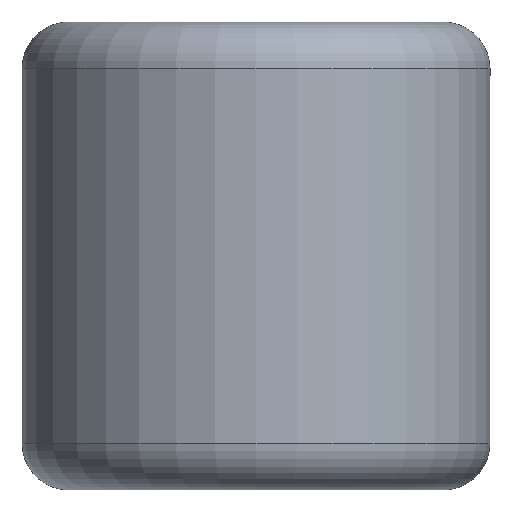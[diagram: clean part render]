
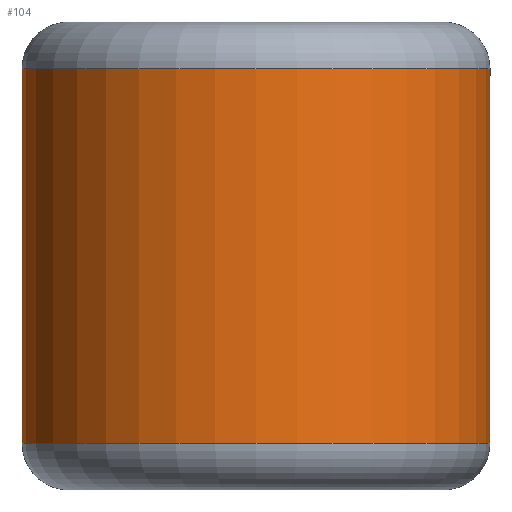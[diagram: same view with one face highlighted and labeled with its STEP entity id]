
A CAD part, left-side view. The second image highlights one B-rep face of the part: STEP entity #104.
In plain terms, the highlighted cylindrical face has radius 5 mm (diameter 10 mm), a partial arc.
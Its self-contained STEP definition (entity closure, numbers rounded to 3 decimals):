
#1 = EDGE_CURVE ( 'NONE', #116, #120, #55, .T. ) ;
#17 = AXIS2_PLACEMENT_3D ( 'NONE', #171, #175, #162 ) ;
#28 = CYLINDRICAL_SURFACE ( 'NONE', #46, 5. ) ;
#30 = EDGE_CURVE ( 'NONE', #116, #189, #185, .T. ) ;
#32 = VECTOR ( 'NONE', #237, 1000. ) ;
#46 = AXIS2_PLACEMENT_3D ( 'NONE', #106, #131, #80 ) ;
#55 = LINE ( 'NONE', #216, #32 ) ;
#56 = EDGE_CURVE ( 'NONE', #110, #120, #75, .T. ) ;
#75 = CIRCLE ( 'NONE', #17, 5. ) ;
#77 = CARTESIAN_POINT ( 'NONE',  ( 0., 10., 4. ) ) ;
#80 = DIRECTION ( 'NONE',  ( 0., 1., 0. ) ) ;
#83 = CARTESIAN_POINT ( 'NONE',  ( 0., 0., -4. ) ) ;
#88 = EDGE_CURVE ( 'NONE', #189, #110, #139, .T. ) ;
#98 = ORIENTED_EDGE ( 'NONE', *, *, #1, .F. ) ;
#100 = ORIENTED_EDGE ( 'NONE', *, *, #56, .T. ) ;
#104 = ADVANCED_FACE ( 'NONE', ( #158 ), #28, .T. ) ;
#106 = CARTESIAN_POINT ( 'NONE',  ( 0., 5., 5. ) ) ;
#109 = DIRECTION ( 'NONE',  ( 0., 0., -1. ) ) ;
#110 = VERTEX_POINT ( 'NONE', #136 ) ;
#114 = ORIENTED_EDGE ( 'NONE', *, *, #30, .T. ) ;
#116 = VERTEX_POINT ( 'NONE', #123 ) ;
#120 = VERTEX_POINT ( 'NONE', #83 ) ;
#123 = CARTESIAN_POINT ( 'NONE',  ( 0., 0., 4. ) ) ;
#127 = CARTESIAN_POINT ( 'NONE',  ( 0., 10., 5. ) ) ;
#131 = DIRECTION ( 'NONE',  ( 0., 0., -1. ) ) ;
#136 = CARTESIAN_POINT ( 'NONE',  ( 0., 10., -4. ) ) ;
#138 = VECTOR ( 'NONE', #109, 1000. ) ;
#139 = LINE ( 'NONE', #127, #138 ) ;
#158 = FACE_OUTER_BOUND ( 'NONE', #239, .T. ) ;
#162 = DIRECTION ( 'NONE',  ( 0., -1., 0. ) ) ;
#171 = CARTESIAN_POINT ( 'NONE',  ( 0., 5., -4. ) ) ;
#175 = DIRECTION ( 'NONE',  ( 0., 0., 1. ) ) ;
#185 = CIRCLE ( 'NONE', #241, 5. ) ;
#189 = VERTEX_POINT ( 'NONE', #77 ) ;
#216 = CARTESIAN_POINT ( 'NONE',  ( 0., 0., 5. ) ) ;
#227 = CARTESIAN_POINT ( 'NONE',  ( 0., 5., 4. ) ) ;
#228 = DIRECTION ( 'NONE',  ( 0., 0., -1. ) ) ;
#229 = ORIENTED_EDGE ( 'NONE', *, *, #88, .T. ) ;
#230 = DIRECTION ( 'NONE',  ( 0., -1., 0. ) ) ;
#237 = DIRECTION ( 'NONE',  ( 0., 0., -1. ) ) ;
#239 = EDGE_LOOP ( 'NONE', ( #98, #114, #229, #100 ) ) ;
#241 = AXIS2_PLACEMENT_3D ( 'NONE', #227, #228, #230 ) ;
